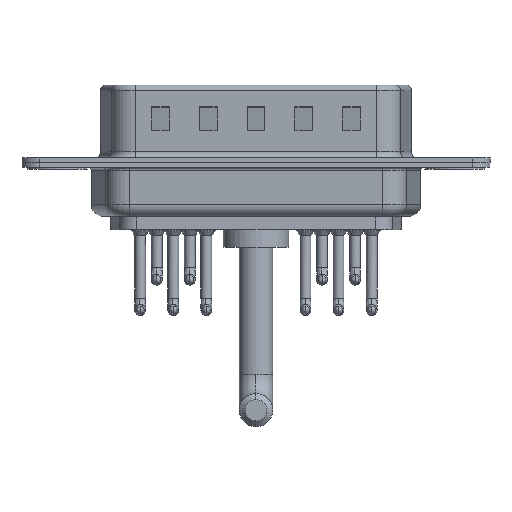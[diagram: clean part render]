
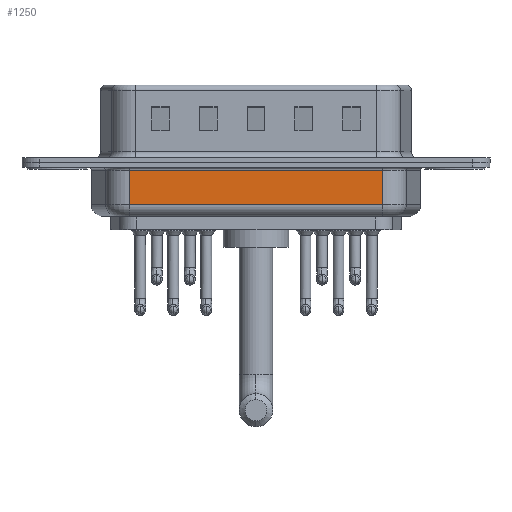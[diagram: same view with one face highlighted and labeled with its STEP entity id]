
A CAD part, front view. The second image highlights one B-rep face of the part: STEP entity #1250.
In plain terms, the highlighted planar face has unit normal (0, -1, 0).
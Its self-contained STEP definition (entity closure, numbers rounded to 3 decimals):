
#11 = VECTOR ( 'NONE', #7451, 1000. ) ;
#517 = DIRECTION ( 'NONE',  ( -1., 0., 0. ) ) ;
#522 = ORIENTED_EDGE ( 'NONE', *, *, #1698, .T. ) ;
#615 = DIRECTION ( 'NONE',  ( 0., 0., 1. ) ) ;
#942 = VERTEX_POINT ( 'NONE', #12028 ) ;
#1250 = ADVANCED_FACE ( 'NONE', ( #16575 ), #2622, .F. ) ;
#1698 = EDGE_CURVE ( 'NONE', #942, #4088, #6976, .T. ) ;
#2078 = VERTEX_POINT ( 'NONE', #12243 ) ;
#2550 = LINE ( 'NONE', #20235, #11 ) ;
#2622 = PLANE ( 'NONE',  #19214 ) ;
#3638 = CARTESIAN_POINT ( 'NONE',  ( 6.031, -5.35, -0.65 ) ) ;
#4088 = VERTEX_POINT ( 'NONE', #16255 ) ;
#4242 = ORIENTED_EDGE ( 'NONE', *, *, #10968, .T. ) ;
#5750 = DIRECTION ( 'NONE',  ( 0., 0., 1. ) ) ;
#6001 = ORIENTED_EDGE ( 'NONE', *, *, #11721, .T. ) ;
#6976 = LINE ( 'NONE', #18316, #19904 ) ;
#7451 = DIRECTION ( 'NONE',  ( 1., 0., 0. ) ) ;
#8355 = CARTESIAN_POINT ( 'NONE',  ( 6.031, -5.35, -3.5 ) ) ;
#8776 = CARTESIAN_POINT ( 'NONE',  ( 6.031, -5.35, -4.5 ) ) ;
#8870 = VERTEX_POINT ( 'NONE', #8355 ) ;
#10283 = LINE ( 'NONE', #12060, #18344 ) ;
#10348 = VECTOR ( 'NONE', #517, 1000. ) ;
#10968 = EDGE_CURVE ( 'NONE', #8870, #942, #2550, .T. ) ;
#11721 = EDGE_CURVE ( 'NONE', #4088, #2078, #19663, .T. ) ;
#12028 = CARTESIAN_POINT ( 'NONE',  ( 27.269, -5.35, -3.5 ) ) ;
#12060 = CARTESIAN_POINT ( 'NONE',  ( 6.031, -5.35, -4.5 ) ) ;
#12243 = CARTESIAN_POINT ( 'NONE',  ( 6.031, -5.35, -0.65 ) ) ;
#13680 = EDGE_CURVE ( 'NONE', #8870, #2078, #10283, .T. ) ;
#16255 = CARTESIAN_POINT ( 'NONE',  ( 27.269, -5.35, -0.65 ) ) ;
#16450 = EDGE_LOOP ( 'NONE', ( #18259, #4242, #522, #6001 ) ) ;
#16575 = FACE_OUTER_BOUND ( 'NONE', #16450, .T. ) ;
#18259 = ORIENTED_EDGE ( 'NONE', *, *, #13680, .F. ) ;
#18316 = CARTESIAN_POINT ( 'NONE',  ( 27.269, -5.35, -4.5 ) ) ;
#18344 = VECTOR ( 'NONE', #18395, 1000. ) ;
#18395 = DIRECTION ( 'NONE',  ( 0., 0., 1. ) ) ;
#19214 = AXIS2_PLACEMENT_3D ( 'NONE', #8776, #19998, #5750 ) ;
#19663 = LINE ( 'NONE', #3638, #10348 ) ;
#19904 = VECTOR ( 'NONE', #615, 1000. ) ;
#19998 = DIRECTION ( 'NONE',  ( 0., 1., 0. ) ) ;
#20235 = CARTESIAN_POINT ( 'NONE',  ( 6.031, -5.35, -3.5 ) ) ;
